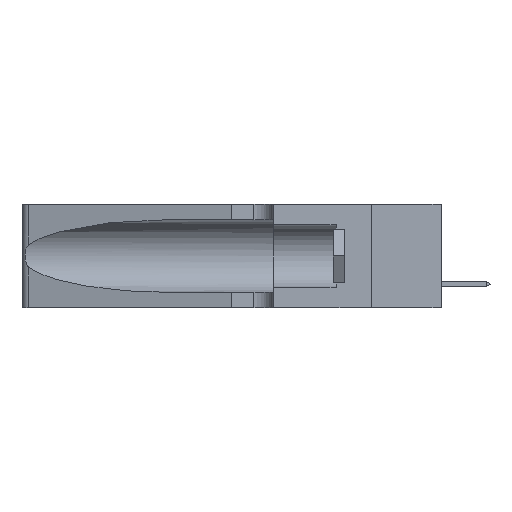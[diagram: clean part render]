
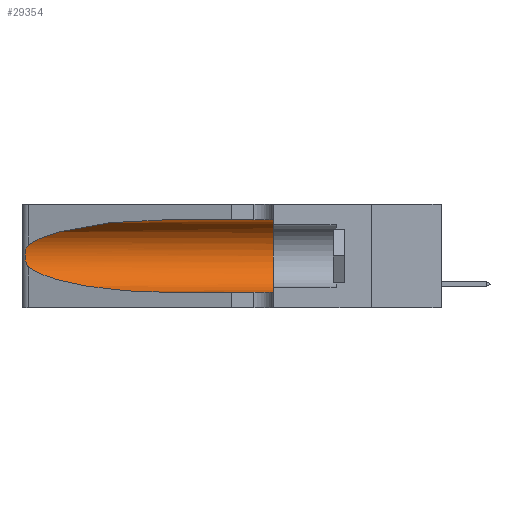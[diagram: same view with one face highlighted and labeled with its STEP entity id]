
A CAD part, left-side view. The second image highlights one B-rep face of the part: STEP entity #29354.
In plain terms, the highlighted cylindrical face has radius 3.308 mm (diameter 6.617 mm), a partial arc.
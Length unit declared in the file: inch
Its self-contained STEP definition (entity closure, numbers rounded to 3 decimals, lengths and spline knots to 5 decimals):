
#75 = EDGE_CURVE ( 'NONE', #25759, #36389, #4253, .T. ) ;
#1659 = DIRECTION ( 'NONE',  ( 0., -1., 0. ) ) ;
#2862 = EDGE_CURVE ( 'NONE', #25759, #4268, #21367, .T. ) ;
#3653 = ORIENTED_EDGE ( 'NONE', *, *, #27765, .T. ) ;
#4253 =( BOUNDED_CURVE ( )  B_SPLINE_CURVE ( 3, ( #10668, #42855, #18299, #11403 ),
 .UNSPECIFIED., .F., .F. ) 
 B_SPLINE_CURVE_WITH_KNOTS ( ( 4, 4 ),
 ( 1.5708, 2.84003 ),
 .UNSPECIFIED. ) 
 CURVE ( )  GEOMETRIC_REPRESENTATION_ITEM ( )  RATIONAL_B_SPLINE_CURVE ( ( 1., 0.87, 0.87, 1. ) ) 
 REPRESENTATION_ITEM ( '' )  );
#4268 = VERTEX_POINT ( 'NONE', #36398 ) ;
#4953 = CARTESIAN_POINT ( 'NONE',  ( 0.25487, 1.22718, 0.22369 ) ) ;
#8567 = CARTESIAN_POINT ( 'NONE',  ( 0.1305, 1.61858, 0.185 ) ) ;
#8790 = CARTESIAN_POINT ( 'NONE',  ( 0.25555, 1.22993, 0.14849 ) ) ;
#9180 = LINE ( 'NONE', #33734, #39922 ) ;
#9468 = CARTESIAN_POINT ( 'NONE',  ( 0.26075, 1.23896, 0.19203 ) ) ;
#9910 = AXIS2_PLACEMENT_3D ( 'NONE', #8567, #41076, #19669 ) ;
#10589 = DIRECTION ( 'NONE',  ( 0., -1., 0. ) ) ;
#10668 = CARTESIAN_POINT ( 'NONE',  ( 0.1305, 0.72297, 0.31525 ) ) ;
#11403 = CARTESIAN_POINT ( 'NONE',  ( 0.25487, 1.22718, 0.22369 ) ) ;
#11618 = ORIENTED_EDGE ( 'NONE', *, *, #21352, .F. ) ;
#13065 = EDGE_LOOP ( 'NONE', ( #37383, #3653, #42917, #35651, #11618, #34052 ) ) ;
#14105 = VECTOR ( 'NONE', #10589, 39.37008 ) ;
#17315 = CARTESIAN_POINT ( 'NONE',  ( 0.1305, 1.61858, 0.31525 ) ) ;
#17449 = CARTESIAN_POINT ( 'NONE',  ( 0.1305, 0.35, 0.05475 ) ) ;
#17741 = DIRECTION ( 'NONE',  ( 0., 1., 0. ) ) ;
#18299 = CARTESIAN_POINT ( 'NONE',  ( 0.2373, 1.15595, 0.28018 ) ) ;
#18835 = B_SPLINE_CURVE_WITH_KNOTS ( 'NONE', 3,
 ( #4953, #29952, #44306, #30589, #41517, #34823, #9468, #44762, #41992, #36016, #43770, #19421, #8790, #30530 ),
 .UNSPECIFIED., .F., .F.,
 ( 4, 2, 2, 2, 2, 2, 4 ),
 ( 0., 0.00027, 0.00053, 0.00107, 0.0016, 0.00187, 0.00214 ),
 .UNSPECIFIED. ) ;
#19421 = CARTESIAN_POINT ( 'NONE',  ( 0.25639, 1.23186, 0.15144 ) ) ;
#19669 = DIRECTION ( 'NONE',  ( 0., 0., -1. ) ) ;
#19702 = AXIS2_PLACEMENT_3D ( 'NONE', #39155, #17741, #35285 ) ;
#20013 = CIRCLE ( 'NONE', #19702, 0.13025 ) ;
#20909 = FACE_OUTER_BOUND ( 'NONE', #13065, .T. ) ;
#21097 = VERTEX_POINT ( 'NONE', #39064 ) ;
#21352 = EDGE_CURVE ( 'NONE', #4268, #40688, #20013, .T. ) ;
#21367 = LINE ( 'NONE', #17315, #14105 ) ;
#22871 = CARTESIAN_POINT ( 'NONE',  ( 0.25487, 1.22718, 0.14631 ) ) ;
#25759 = VERTEX_POINT ( 'NONE', #45665 ) ;
#26118 = CARTESIAN_POINT ( 'NONE',  ( 0.2373, 1.15595, 0.08982 ) ) ;
#27765 = EDGE_CURVE ( 'NONE', #36389, #30405, #18835, .T. ) ;
#29107 = EDGE_CURVE ( 'NONE', #21097, #40688, #9180, .T. ) ;
#29220 = CYLINDRICAL_SURFACE ( 'NONE', #9910, 0.13025 ) ;
#29354 = ADVANCED_FACE ( 'NONE', ( #20909 ), #29220, .F. ) ;
#29952 = CARTESIAN_POINT ( 'NONE',  ( 0.25555, 1.22994, 0.2215 ) ) ;
#30405 = VERTEX_POINT ( 'NONE', #42156 ) ;
#30530 = CARTESIAN_POINT ( 'NONE',  ( 0.25487, 1.22718, 0.14631 ) ) ;
#30589 = CARTESIAN_POINT ( 'NONE',  ( 0.25787, 1.23484, 0.2124 ) ) ;
#30680 = CARTESIAN_POINT ( 'NONE',  ( 0.18966, 0.96281, 0.05475 ) ) ;
#33734 = CARTESIAN_POINT ( 'NONE',  ( 0.1305, 1.61858, 0.05475 ) ) ;
#34052 = ORIENTED_EDGE ( 'NONE', *, *, #2862, .F. ) ;
#34823 = CARTESIAN_POINT ( 'NONE',  ( 0.26018, 1.23835, 0.19895 ) ) ;
#35285 = DIRECTION ( 'NONE',  ( 0., 0., 1. ) ) ;
#35651 = ORIENTED_EDGE ( 'NONE', *, *, #29107, .T. ) ;
#35677 = EDGE_CURVE ( 'NONE', #30405, #21097, #41792, .T. ) ;
#36016 = CARTESIAN_POINT ( 'NONE',  ( 0.25856, 1.23593, 0.16098 ) ) ;
#36389 = VERTEX_POINT ( 'NONE', #37233 ) ;
#36398 = CARTESIAN_POINT ( 'NONE',  ( 0.1305, 0.35, 0.31525 ) ) ;
#37233 = CARTESIAN_POINT ( 'NONE',  ( 0.25487, 1.22718, 0.22369 ) ) ;
#37383 = ORIENTED_EDGE ( 'NONE', *, *, #75, .T. ) ;
#38026 = CARTESIAN_POINT ( 'NONE',  ( 0.1305, 0.72297, 0.05475 ) ) ;
#39064 = CARTESIAN_POINT ( 'NONE',  ( 0.1305, 0.72297, 0.05475 ) ) ;
#39155 = CARTESIAN_POINT ( 'NONE',  ( 0.1305, 0.35, 0.185 ) ) ;
#39922 = VECTOR ( 'NONE', #1659, 39.37008 ) ;
#40688 = VERTEX_POINT ( 'NONE', #17449 ) ;
#41076 = DIRECTION ( 'NONE',  ( 0., -1., 0. ) ) ;
#41517 = CARTESIAN_POINT ( 'NONE',  ( 0.25854, 1.2359, 0.20912 ) ) ;
#41792 =( BOUNDED_CURVE ( )  B_SPLINE_CURVE ( 3, ( #22871, #26118, #30680, #38026 ),
 .UNSPECIFIED., .F., .T. ) 
 B_SPLINE_CURVE_WITH_KNOTS ( ( 4, 4 ),
 ( 3.44316, 4.71239 ),
 .UNSPECIFIED. ) 
 CURVE ( )  GEOMETRIC_REPRESENTATION_ITEM ( )  RATIONAL_B_SPLINE_CURVE ( ( 1., 0.87, 0.87, 1. ) ) 
 REPRESENTATION_ITEM ( '' )  );
#41992 = CARTESIAN_POINT ( 'NONE',  ( 0.26017, 1.23833, 0.17102 ) ) ;
#42156 = CARTESIAN_POINT ( 'NONE',  ( 0.25487, 1.22718, 0.14631 ) ) ;
#42855 = CARTESIAN_POINT ( 'NONE',  ( 0.18966, 0.96281, 0.31525 ) ) ;
#42917 = ORIENTED_EDGE ( 'NONE', *, *, #35677, .T. ) ;
#43770 = CARTESIAN_POINT ( 'NONE',  ( 0.25789, 1.23486, 0.15765 ) ) ;
#44306 = CARTESIAN_POINT ( 'NONE',  ( 0.25639, 1.23184, 0.21858 ) ) ;
#44762 = CARTESIAN_POINT ( 'NONE',  ( 0.26075, 1.23896, 0.178 ) ) ;
#45665 = CARTESIAN_POINT ( 'NONE',  ( 0.1305, 0.72297, 0.31525 ) ) ;
